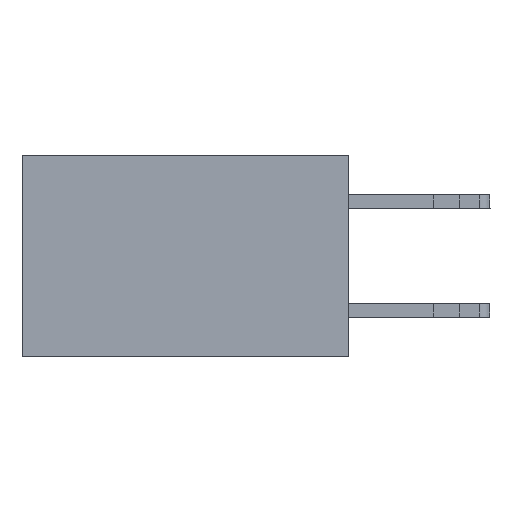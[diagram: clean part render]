
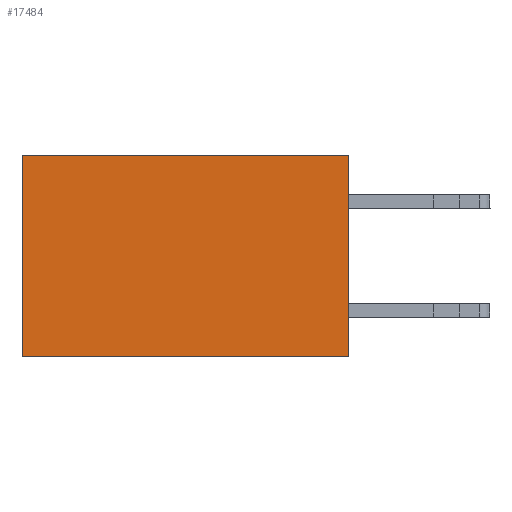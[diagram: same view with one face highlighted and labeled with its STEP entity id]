
A CAD part, left-side view. The second image highlights one B-rep face of the part: STEP entity #17484.
In plain terms, the highlighted planar face has unit normal (-1, 0, 0).
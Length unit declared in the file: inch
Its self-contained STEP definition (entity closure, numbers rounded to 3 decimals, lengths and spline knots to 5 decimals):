
#116 = CARTESIAN_POINT ( 'NONE',  ( 0.2615, 0.6, -0.37 ) ) ;
#217 = DIRECTION ( 'NONE',  ( 0., 0., -1. ) ) ;
#3475 = EDGE_CURVE ( 'NONE', #4522, #21360, #15965, .T. ) ;
#4100 = LINE ( 'NONE', #14879, #12759 ) ;
#4522 = VERTEX_POINT ( 'NONE', #10917 ) ;
#4985 = ORIENTED_EDGE ( 'NONE', *, *, #3475, .T. ) ;
#5428 = CARTESIAN_POINT ( 'NONE',  ( 0.2615, 0.6, -0.37 ) ) ;
#5586 = EDGE_CURVE ( 'NONE', #21360, #9943, #17567, .T. ) ;
#5791 = PLANE ( 'NONE',  #19481 ) ;
#5894 = EDGE_LOOP ( 'NONE', ( #14972, #12712, #13965, #4985 ) ) ;
#6394 = DIRECTION ( 'NONE',  ( 0., 0., -1. ) ) ;
#6438 = VERTEX_POINT ( 'NONE', #15500 ) ;
#6545 = CARTESIAN_POINT ( 'NONE',  ( 0.2615, 0., -0.37 ) ) ;
#6915 = VECTOR ( 'NONE', #6394, 39.37008 ) ;
#7736 = FACE_OUTER_BOUND ( 'NONE', #5894, .T. ) ;
#9302 = CARTESIAN_POINT ( 'NONE',  ( 0.2615, 0., -0.37 ) ) ;
#9943 = VERTEX_POINT ( 'NONE', #5428 ) ;
#10028 = CARTESIAN_POINT ( 'NONE',  ( 0.2615, 0.6, 0. ) ) ;
#10917 = CARTESIAN_POINT ( 'NONE',  ( 0.2615, 0., 0. ) ) ;
#10980 = VECTOR ( 'NONE', #15973, 39.37008 ) ;
#11049 = DIRECTION ( 'NONE',  ( 0., 0., -1. ) ) ;
#11136 = EDGE_CURVE ( 'NONE', #4522, #6438, #12040, .T. ) ;
#12040 = LINE ( 'NONE', #6545, #6915 ) ;
#12712 = ORIENTED_EDGE ( 'NONE', *, *, #13292, .F. ) ;
#12759 = VECTOR ( 'NONE', #18235, 39.37008 ) ;
#13292 = EDGE_CURVE ( 'NONE', #6438, #9943, #4100, .T. ) ;
#13965 = ORIENTED_EDGE ( 'NONE', *, *, #11136, .F. ) ;
#14509 = CARTESIAN_POINT ( 'NONE',  ( 0.2615, 0., 0. ) ) ;
#14879 = CARTESIAN_POINT ( 'NONE',  ( 0.2615, 0., -0.37 ) ) ;
#14972 = ORIENTED_EDGE ( 'NONE', *, *, #5586, .T. ) ;
#15500 = CARTESIAN_POINT ( 'NONE',  ( 0.2615, 0., -0.37 ) ) ;
#15965 = LINE ( 'NONE', #14509, #10980 ) ;
#15973 = DIRECTION ( 'NONE',  ( 0., 1., 0. ) ) ;
#17484 = ADVANCED_FACE ( 'NONE', ( #7736 ), #5791, .F. ) ;
#17567 = LINE ( 'NONE', #116, #20393 ) ;
#18235 = DIRECTION ( 'NONE',  ( 0., 1., 0. ) ) ;
#19481 = AXIS2_PLACEMENT_3D ( 'NONE', #9302, #21004, #11049 ) ;
#20393 = VECTOR ( 'NONE', #217, 39.37008 ) ;
#21004 = DIRECTION ( 'NONE',  ( 1., 0., 0. ) ) ;
#21360 = VERTEX_POINT ( 'NONE', #10028 ) ;
